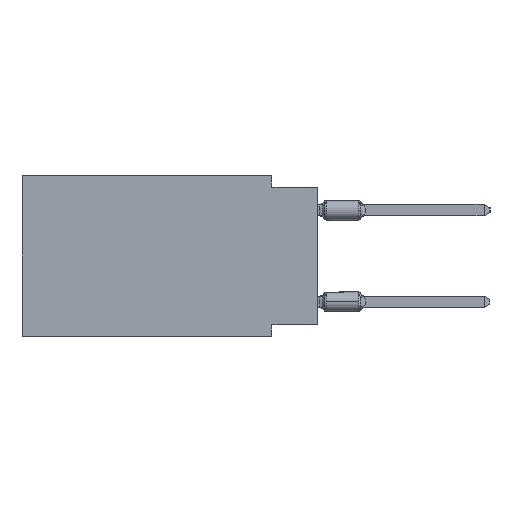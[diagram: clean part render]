
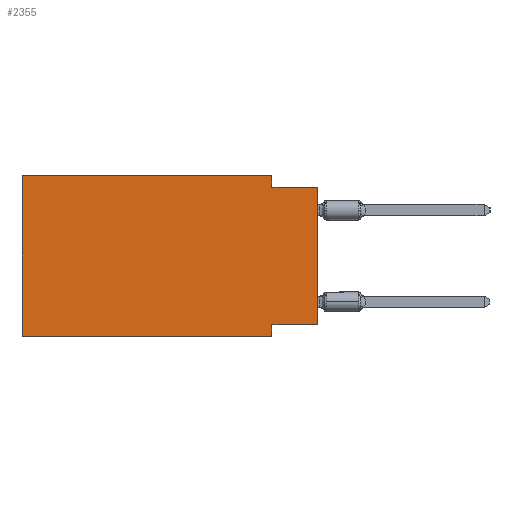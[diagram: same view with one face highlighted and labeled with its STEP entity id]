
A CAD part, left-side view. The second image highlights one B-rep face of the part: STEP entity #2355.
In plain terms, the highlighted planar face has unit normal (-1, 0, 0).
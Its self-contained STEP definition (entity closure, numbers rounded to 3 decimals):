
#11 = EDGE_CURVE ( 'NONE', #23577, #1656, #13921, .T. ) ;
#130 = AXIS2_PLACEMENT_3D ( 'NONE', #27727, #8946, #33519 ) ;
#1656 = VERTEX_POINT ( 'NONE', #20030 ) ;
#1793 = CARTESIAN_POINT ( 'NONE',  ( 0., 2.54, -8.89 ) ) ;
#2037 = CARTESIAN_POINT ( 'NONE',  ( 0., 16.383, -8.89 ) ) ;
#2083 = VECTOR ( 'NONE', #26414, 1000. ) ;
#2297 = ORIENTED_EDGE ( 'NONE', *, *, #30306, .F. ) ;
#2355 = ADVANCED_FACE ( 'NONE', ( #7673 ), #3520, .F. ) ;
#2497 = LINE ( 'NONE', #1793, #25728 ) ;
#3032 = CARTESIAN_POINT ( 'NONE',  ( 0., 2.54, -8.255 ) ) ;
#3520 = PLANE ( 'NONE',  #130 ) ;
#5034 = DIRECTION ( 'NONE',  ( 0., 0., -1. ) ) ;
#5398 = VECTOR ( 'NONE', #27140, 1000. ) ;
#6375 = EDGE_CURVE ( 'NONE', #1656, #28572, #7430, .T. ) ;
#7430 = LINE ( 'NONE', #29476, #2083 ) ;
#7673 = FACE_OUTER_BOUND ( 'NONE', #15296, .T. ) ;
#7700 = CARTESIAN_POINT ( 'NONE',  ( 0., 2.54, -0.635 ) ) ;
#7847 = VECTOR ( 'NONE', #20492, 1000. ) ;
#7939 = ORIENTED_EDGE ( 'NONE', *, *, #25196, .F. ) ;
#8282 = VERTEX_POINT ( 'NONE', #7700 ) ;
#8946 = DIRECTION ( 'NONE',  ( 1., 0., 0. ) ) ;
#9643 = CARTESIAN_POINT ( 'NONE',  ( 0., 2.54, 0. ) ) ;
#10098 = LINE ( 'NONE', #28720, #17448 ) ;
#11222 = CARTESIAN_POINT ( 'NONE',  ( 0., 16.383, 0. ) ) ;
#11588 = DIRECTION ( 'NONE',  ( 0., 0., 1. ) ) ;
#12159 = ORIENTED_EDGE ( 'NONE', *, *, #6375, .F. ) ;
#13921 = LINE ( 'NONE', #11222, #18227 ) ;
#14367 = LINE ( 'NONE', #25390, #30981 ) ;
#14971 = DIRECTION ( 'NONE',  ( 0., 0., -1. ) ) ;
#15296 = EDGE_LOOP ( 'NONE', ( #20020, #2297, #23337, #12159, #17193, #20538, #22408, #7939 ) ) ;
#15769 = CARTESIAN_POINT ( 'NONE',  ( 0., 0., -8.255 ) ) ;
#17145 = CARTESIAN_POINT ( 'NONE',  ( 0., 0., -0.635 ) ) ;
#17193 = ORIENTED_EDGE ( 'NONE', *, *, #11, .F. ) ;
#17448 = VECTOR ( 'NONE', #14971, 1000. ) ;
#17737 = EDGE_CURVE ( 'NONE', #23577, #19900, #32920, .T. ) ;
#18227 = VECTOR ( 'NONE', #11588, 1000. ) ;
#19670 = LINE ( 'NONE', #17145, #23596 ) ;
#19900 = VERTEX_POINT ( 'NONE', #33199 ) ;
#20020 = ORIENTED_EDGE ( 'NONE', *, *, #34059, .T. ) ;
#20030 = CARTESIAN_POINT ( 'NONE',  ( 0., 16.383, 0. ) ) ;
#20492 = DIRECTION ( 'NONE',  ( 0., 0., 1. ) ) ;
#20538 = ORIENTED_EDGE ( 'NONE', *, *, #17737, .T. ) ;
#20836 = EDGE_CURVE ( 'NONE', #28572, #8282, #10098, .T. ) ;
#22408 = ORIENTED_EDGE ( 'NONE', *, *, #31852, .F. ) ;
#23014 = VERTEX_POINT ( 'NONE', #25646 ) ;
#23337 = ORIENTED_EDGE ( 'NONE', *, *, #20836, .F. ) ;
#23577 = VERTEX_POINT ( 'NONE', #23768 ) ;
#23596 = VECTOR ( 'NONE', #30170, 1000. ) ;
#23768 = CARTESIAN_POINT ( 'NONE',  ( 0., 16.383, -8.89 ) ) ;
#24701 = VERTEX_POINT ( 'NONE', #3032 ) ;
#25196 = EDGE_CURVE ( 'NONE', #25867, #24701, #14367, .T. ) ;
#25390 = CARTESIAN_POINT ( 'NONE',  ( 0., 0., -8.255 ) ) ;
#25646 = CARTESIAN_POINT ( 'NONE',  ( 0., 0., -0.635 ) ) ;
#25728 = VECTOR ( 'NONE', #5034, 1000. ) ;
#25867 = VERTEX_POINT ( 'NONE', #15769 ) ;
#26414 = DIRECTION ( 'NONE',  ( 0., -1., 0. ) ) ;
#27140 = DIRECTION ( 'NONE',  ( 0., -1., 0. ) ) ;
#27727 = CARTESIAN_POINT ( 'NONE',  ( 0., 16.383, 0. ) ) ;
#27926 = LINE ( 'NONE', #31538, #7847 ) ;
#28453 = DIRECTION ( 'NONE',  ( 0., 1., 0. ) ) ;
#28572 = VERTEX_POINT ( 'NONE', #9643 ) ;
#28720 = CARTESIAN_POINT ( 'NONE',  ( 0., 2.54, 0. ) ) ;
#29476 = CARTESIAN_POINT ( 'NONE',  ( 0., 16.383, 0. ) ) ;
#30170 = DIRECTION ( 'NONE',  ( 0., -1., 0. ) ) ;
#30306 = EDGE_CURVE ( 'NONE', #8282, #23014, #19670, .T. ) ;
#30981 = VECTOR ( 'NONE', #28453, 1000. ) ;
#31538 = CARTESIAN_POINT ( 'NONE',  ( 0., 0., 0. ) ) ;
#31852 = EDGE_CURVE ( 'NONE', #24701, #19900, #2497, .T. ) ;
#32920 = LINE ( 'NONE', #2037, #5398 ) ;
#33199 = CARTESIAN_POINT ( 'NONE',  ( 0., 2.54, -8.89 ) ) ;
#33519 = DIRECTION ( 'NONE',  ( 0., 0., -1. ) ) ;
#34059 = EDGE_CURVE ( 'NONE', #25867, #23014, #27926, .T. ) ;
